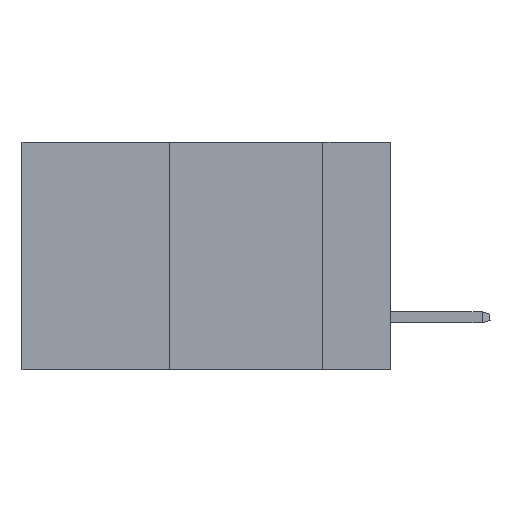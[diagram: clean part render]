
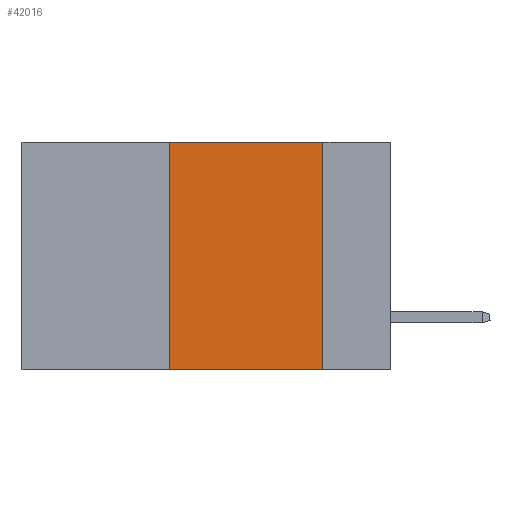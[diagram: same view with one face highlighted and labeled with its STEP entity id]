
A CAD part, left-side view. The second image highlights one B-rep face of the part: STEP entity #42016.
In plain terms, the highlighted planar face has unit normal (-1, 0, 0).
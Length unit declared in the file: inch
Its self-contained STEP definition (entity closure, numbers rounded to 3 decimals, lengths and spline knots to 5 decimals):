
#288 = LINE ( 'NONE', #11278, #45915 ) ;
#1291 = CARTESIAN_POINT ( 'NONE',  ( 0., 0.6, 0. ) ) ;
#3688 = EDGE_CURVE ( 'NONE', #16050, #40673, #8668, .T. ) ;
#3995 = VECTOR ( 'NONE', #44010, 39.37008 ) ;
#4928 = DIRECTION ( 'NONE',  ( 0., -1., 0. ) ) ;
#5219 = PLANE ( 'NONE',  #39872 ) ;
#7043 = VECTOR ( 'NONE', #4928, 39.37008 ) ;
#7772 = EDGE_CURVE ( 'NONE', #46258, #40673, #16136, .T. ) ;
#8668 = LINE ( 'NONE', #20993, #13359 ) ;
#9645 = CARTESIAN_POINT ( 'NONE',  ( 0., 0.6, 0. ) ) ;
#10632 = CARTESIAN_POINT ( 'NONE',  ( 0., 0.36, -0.37 ) ) ;
#11278 = CARTESIAN_POINT ( 'NONE',  ( 0., 0.36, 0. ) ) ;
#12751 = CARTESIAN_POINT ( 'NONE',  ( 0., 0.6, -0.37 ) ) ;
#13359 = VECTOR ( 'NONE', #40688, 39.37008 ) ;
#14338 = LINE ( 'NONE', #9645, #3995 ) ;
#15326 = FACE_OUTER_BOUND ( 'NONE', #18687, .T. ) ;
#16050 = VERTEX_POINT ( 'NONE', #49721 ) ;
#16136 = LINE ( 'NONE', #12751, #7043 ) ;
#18687 = EDGE_LOOP ( 'NONE', ( #25053, #49869, #44374, #37999 ) ) ;
#20993 = CARTESIAN_POINT ( 'NONE',  ( 0., 0.11, 0. ) ) ;
#21006 = DIRECTION ( 'NONE',  ( 1., 0., 0. ) ) ;
#22464 = EDGE_CURVE ( 'NONE', #46258, #45765, #288, .T. ) ;
#25053 = ORIENTED_EDGE ( 'NONE', *, *, #3688, .F. ) ;
#32362 = DIRECTION ( 'NONE',  ( 0., 0., -1. ) ) ;
#33332 = DIRECTION ( 'NONE',  ( 0., 0., 1. ) ) ;
#35299 = EDGE_CURVE ( 'NONE', #45765, #16050, #14338, .T. ) ;
#37999 = ORIENTED_EDGE ( 'NONE', *, *, #7772, .T. ) ;
#38874 = CARTESIAN_POINT ( 'NONE',  ( 0., 0.11, -0.37 ) ) ;
#38897 = CARTESIAN_POINT ( 'NONE',  ( 0., 0.36, 0. ) ) ;
#39872 = AXIS2_PLACEMENT_3D ( 'NONE', #1291, #21006, #32362 ) ;
#40673 = VERTEX_POINT ( 'NONE', #38874 ) ;
#40688 = DIRECTION ( 'NONE',  ( 0., 0., -1. ) ) ;
#42016 = ADVANCED_FACE ( 'NONE', ( #15326 ), #5219, .F. ) ;
#44010 = DIRECTION ( 'NONE',  ( 0., -1., 0. ) ) ;
#44374 = ORIENTED_EDGE ( 'NONE', *, *, #22464, .F. ) ;
#45765 = VERTEX_POINT ( 'NONE', #38897 ) ;
#45915 = VECTOR ( 'NONE', #33332, 39.37008 ) ;
#46258 = VERTEX_POINT ( 'NONE', #10632 ) ;
#49721 = CARTESIAN_POINT ( 'NONE',  ( 0., 0.11, 0. ) ) ;
#49869 = ORIENTED_EDGE ( 'NONE', *, *, #35299, .F. ) ;
